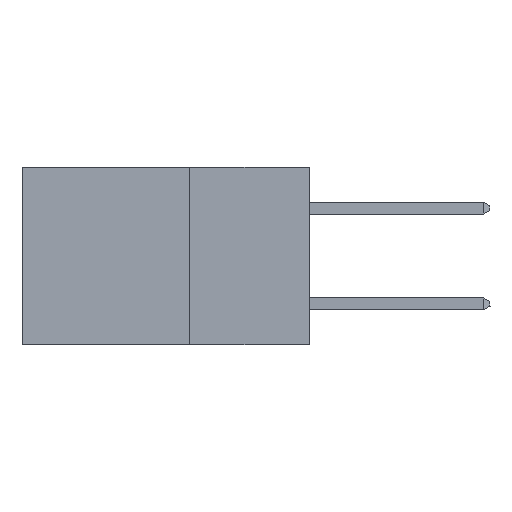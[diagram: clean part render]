
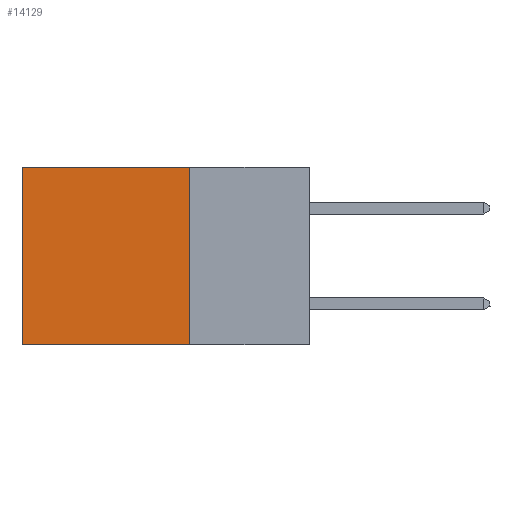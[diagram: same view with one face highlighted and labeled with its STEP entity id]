
A CAD part, left-side view. The second image highlights one B-rep face of the part: STEP entity #14129.
In plain terms, the highlighted planar face has unit normal (-1, 0, 0).
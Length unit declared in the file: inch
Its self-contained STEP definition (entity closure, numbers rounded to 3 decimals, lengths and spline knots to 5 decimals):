
#1470 = PLANE ( 'NONE',  #16445 ) ;
#2079 = ORIENTED_EDGE ( 'NONE', *, *, #2751, .F. ) ;
#2153 = EDGE_CURVE ( 'NONE', #7861, #11381, #11491, .T. ) ;
#2751 = EDGE_CURVE ( 'NONE', #15457, #11761, #15715, .T. ) ;
#3624 = FACE_OUTER_BOUND ( 'NONE', #3931, .T. ) ;
#3644 = CARTESIAN_POINT ( 'NONE',  ( 0.2875, 0.6, 0. ) ) ;
#3931 = EDGE_LOOP ( 'NONE', ( #9314, #12328, #2079, #6653 ) ) ;
#4235 = DIRECTION ( 'NONE',  ( 0., 0., -1. ) ) ;
#4885 = CARTESIAN_POINT ( 'NONE',  ( 0.2875, 0.6, -0.37 ) ) ;
#6653 = ORIENTED_EDGE ( 'NONE', *, *, #16700, .T. ) ;
#6996 = VECTOR ( 'NONE', #13244, 39.37008 ) ;
#7861 = VERTEX_POINT ( 'NONE', #22458 ) ;
#9137 = CARTESIAN_POINT ( 'NONE',  ( 0.2875, 0.25, -0.37 ) ) ;
#9314 = ORIENTED_EDGE ( 'NONE', *, *, #2153, .T. ) ;
#11262 = CARTESIAN_POINT ( 'NONE',  ( 0.2875, 0.25, 0. ) ) ;
#11348 = DIRECTION ( 'NONE',  ( 1., 0., 0. ) ) ;
#11381 = VERTEX_POINT ( 'NONE', #4885 ) ;
#11491 = LINE ( 'NONE', #3644, #6996 ) ;
#11761 = VERTEX_POINT ( 'NONE', #23551 ) ;
#12328 = ORIENTED_EDGE ( 'NONE', *, *, #22642, .F. ) ;
#12642 = VECTOR ( 'NONE', #4235, 39.37008 ) ;
#13030 = LINE ( 'NONE', #9137, #15988 ) ;
#13244 = DIRECTION ( 'NONE',  ( 0., 0., -1. ) ) ;
#13283 = DIRECTION ( 'NONE',  ( 0., 1., 0. ) ) ;
#13707 = CARTESIAN_POINT ( 'NONE',  ( 0.2875, 0.25, 0. ) ) ;
#14129 = ADVANCED_FACE ( 'NONE', ( #3624 ), #1470, .F. ) ;
#15023 = VECTOR ( 'NONE', #16794, 39.37008 ) ;
#15457 = VERTEX_POINT ( 'NONE', #17133 ) ;
#15715 = LINE ( 'NONE', #13707, #12642 ) ;
#15988 = VECTOR ( 'NONE', #13283, 39.37008 ) ;
#16445 = AXIS2_PLACEMENT_3D ( 'NONE', #22683, #11348, #17004 ) ;
#16700 = EDGE_CURVE ( 'NONE', #15457, #7861, #17045, .T. ) ;
#16794 = DIRECTION ( 'NONE',  ( 0., 1., 0. ) ) ;
#17004 = DIRECTION ( 'NONE',  ( 0., 0., -1. ) ) ;
#17045 = LINE ( 'NONE', #11262, #15023 ) ;
#17133 = CARTESIAN_POINT ( 'NONE',  ( 0.2875, 0.25, 0. ) ) ;
#22458 = CARTESIAN_POINT ( 'NONE',  ( 0.2875, 0.6, 0. ) ) ;
#22642 = EDGE_CURVE ( 'NONE', #11761, #11381, #13030, .T. ) ;
#22683 = CARTESIAN_POINT ( 'NONE',  ( 0.2875, 0.25, 0. ) ) ;
#23551 = CARTESIAN_POINT ( 'NONE',  ( 0.2875, 0.25, -0.37 ) ) ;
